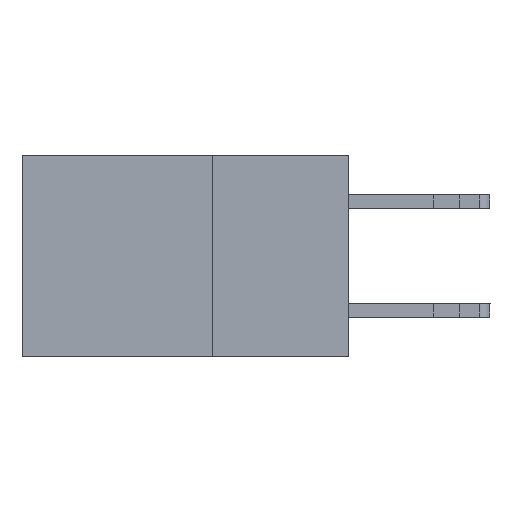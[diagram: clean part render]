
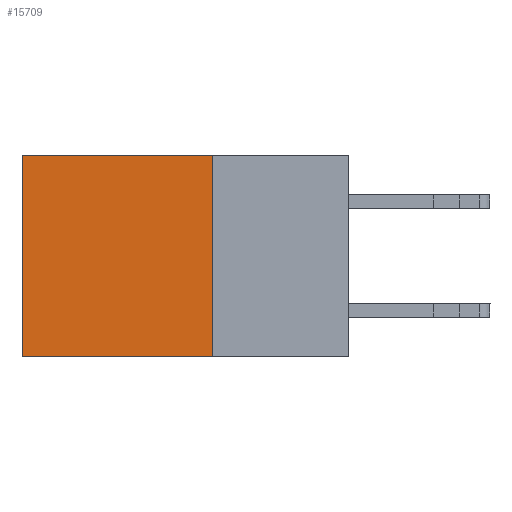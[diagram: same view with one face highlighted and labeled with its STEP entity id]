
A CAD part, left-side view. The second image highlights one B-rep face of the part: STEP entity #15709.
In plain terms, the highlighted planar face has unit normal (-1, 0, 0).
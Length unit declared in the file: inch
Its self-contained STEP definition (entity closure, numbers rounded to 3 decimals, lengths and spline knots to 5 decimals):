
#591 = CARTESIAN_POINT ( 'NONE',  ( 0.2615, 0.25, -0.37 ) ) ;
#1726 = EDGE_CURVE ( 'NONE', #13383, #4428, #19333, .T. ) ;
#1801 = ORIENTED_EDGE ( 'NONE', *, *, #1726, .F. ) ;
#1865 = VECTOR ( 'NONE', #14048, 39.37008 ) ;
#2373 = CARTESIAN_POINT ( 'NONE',  ( 0.2615, 0.6, -0.37 ) ) ;
#3574 = ORIENTED_EDGE ( 'NONE', *, *, #10965, .T. ) ;
#4428 = VERTEX_POINT ( 'NONE', #5420 ) ;
#4929 = VERTEX_POINT ( 'NONE', #10071 ) ;
#5113 = VECTOR ( 'NONE', #7021, 39.37008 ) ;
#5312 = CARTESIAN_POINT ( 'NONE',  ( 0.2615, 0.25, 0. ) ) ;
#5331 = LINE ( 'NONE', #2373, #18838 ) ;
#5420 = CARTESIAN_POINT ( 'NONE',  ( 0.2615, 0.6, -0.37 ) ) ;
#5609 = ORIENTED_EDGE ( 'NONE', *, *, #12780, .T. ) ;
#5755 = PLANE ( 'NONE',  #20555 ) ;
#7021 = DIRECTION ( 'NONE',  ( 0., 1., 0. ) ) ;
#7180 = DIRECTION ( 'NONE',  ( 0., 1., 0. ) ) ;
#7465 = DIRECTION ( 'NONE',  ( 1., 0., 0. ) ) ;
#9119 = EDGE_CURVE ( 'NONE', #14691, #13383, #15388, .T. ) ;
#10071 = CARTESIAN_POINT ( 'NONE',  ( 0.2615, 0.6, 0. ) ) ;
#10965 = EDGE_CURVE ( 'NONE', #14691, #4929, #18641, .T. ) ;
#12599 = CARTESIAN_POINT ( 'NONE',  ( 0.2615, 0.25, -0.37 ) ) ;
#12780 = EDGE_CURVE ( 'NONE', #4929, #4428, #5331, .T. ) ;
#13383 = VERTEX_POINT ( 'NONE', #17264 ) ;
#14048 = DIRECTION ( 'NONE',  ( 0., 0., -1. ) ) ;
#14246 = DIRECTION ( 'NONE',  ( 0., 0., -1. ) ) ;
#14691 = VERTEX_POINT ( 'NONE', #17213 ) ;
#15388 = LINE ( 'NONE', #19063, #1865 ) ;
#15709 = ADVANCED_FACE ( 'NONE', ( #17393 ), #5755, .F. ) ;
#15743 = EDGE_LOOP ( 'NONE', ( #5609, #1801, #18380, #3574 ) ) ;
#17213 = CARTESIAN_POINT ( 'NONE',  ( 0.2615, 0.25, 0. ) ) ;
#17264 = CARTESIAN_POINT ( 'NONE',  ( 0.2615, 0.25, -0.37 ) ) ;
#17393 = FACE_OUTER_BOUND ( 'NONE', #15743, .T. ) ;
#18380 = ORIENTED_EDGE ( 'NONE', *, *, #9119, .F. ) ;
#18641 = LINE ( 'NONE', #5312, #5113 ) ;
#18815 = VECTOR ( 'NONE', #7180, 39.37008 ) ;
#18838 = VECTOR ( 'NONE', #14246, 39.37008 ) ;
#19063 = CARTESIAN_POINT ( 'NONE',  ( 0.2615, 0.25, -0.37 ) ) ;
#19291 = DIRECTION ( 'NONE',  ( 0., 0., -1. ) ) ;
#19333 = LINE ( 'NONE', #12599, #18815 ) ;
#20555 = AXIS2_PLACEMENT_3D ( 'NONE', #591, #7465, #19291 ) ;
